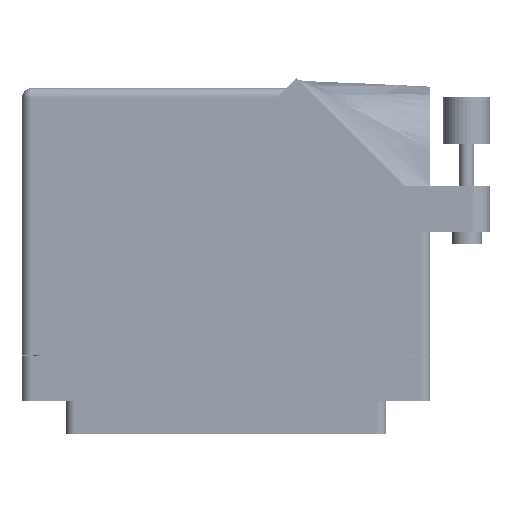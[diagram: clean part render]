
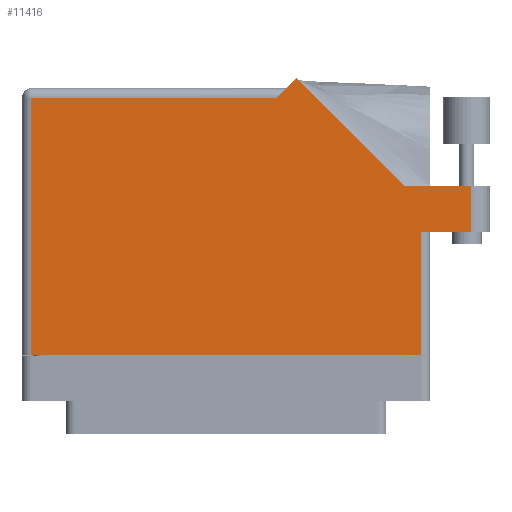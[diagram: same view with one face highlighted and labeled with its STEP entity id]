
A CAD part, front view. The second image highlights one B-rep face of the part: STEP entity #11416.
In plain terms, the highlighted face is planar.
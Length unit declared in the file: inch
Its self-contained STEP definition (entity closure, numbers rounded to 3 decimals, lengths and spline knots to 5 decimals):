
#575 = CARTESIAN_POINT ( 'NONE',  ( 1.297, 0.715, 0.617 ) ) ;
#793 = DIRECTION ( 'NONE',  ( -1., 0., 0. ) ) ;
#1383 = VERTEX_POINT ( 'NONE', #56044 ) ;
#2882 = EDGE_CURVE ( 'NONE', #39727, #57878, #27326, .T. ) ;
#3471 = ORIENTED_EDGE ( 'NONE', *, *, #36136, .T. ) ;
#3594 = VERTEX_POINT ( 'NONE', #21968 ) ;
#4617 = LINE ( 'NONE', #35553, #37606 ) ;
#5000 = DIRECTION ( 'NONE',  ( -1., 0., 0. ) ) ;
#7629 = CARTESIAN_POINT ( 'NONE',  ( -1.297, -0.1, 0.617 ) ) ;
#8923 = CARTESIAN_POINT ( 'NONE',  ( 1.19342, 1.022, 0.617 ) ) ;
#11416 = ADVANCED_FACE ( 'NONE', ( #44479 ), #49639, .F. ) ;
#13056 = VECTOR ( 'NONE', #793, 39.37008 ) ;
#13113 = LINE ( 'NONE', #18179, #72159 ) ;
#14040 = EDGE_CURVE ( 'NONE', #65003, #15289, #53946, .T. ) ;
#14169 = ORIENTED_EDGE ( 'NONE', *, *, #66457, .T. ) ;
#14201 = CARTESIAN_POINT ( 'NONE',  ( 1.297, 0.715, 0.617 ) ) ;
#15011 = CARTESIAN_POINT ( 'NONE',  ( 0.399, 1.675, 0.617 ) ) ;
#15289 = VERTEX_POINT ( 'NONE', #29542 ) ;
#16509 = ORIENTED_EDGE ( 'NONE', *, *, #23540, .T. ) ;
#18179 = CARTESIAN_POINT ( 'NONE',  ( -1.359, -0.1, 0.617 ) ) ;
#18194 = ORIENTED_EDGE ( 'NONE', *, *, #22297, .T. ) ;
#18406 = CARTESIAN_POINT ( 'NONE',  ( 1.759, 1.022, 0.617 ) ) ;
#19467 = CARTESIAN_POINT ( 'NONE',  ( 1.634, 0.715, 0.617 ) ) ;
#19882 = EDGE_LOOP ( 'NONE', ( #3471, #60425, #14169, #16509, #44811, #64625, #18194, #25845, #32673 ) ) ;
#21968 = CARTESIAN_POINT ( 'NONE',  ( 0.337, 1.613, 0.617 ) ) ;
#22297 = EDGE_CURVE ( 'NONE', #1383, #32161, #22574, .T. ) ;
#22574 = LINE ( 'NONE', #53452, #25234 ) ;
#22772 = CARTESIAN_POINT ( 'NONE',  ( 1.297, -0.1, 0.617 ) ) ;
#23540 = EDGE_CURVE ( 'NONE', #53965, #62565, #59020, .T. ) ;
#25234 = VECTOR ( 'NONE', #32179, 39.37008 ) ;
#25845 = ORIENTED_EDGE ( 'NONE', *, *, #62124, .T. ) ;
#26243 = DIRECTION ( 'NONE',  ( 1., 0., 0. ) ) ;
#26257 = VECTOR ( 'NONE', #28335, 39.37008 ) ;
#26466 = VECTOR ( 'NONE', #31413, 39.37008 ) ;
#27132 = CARTESIAN_POINT ( 'NONE',  ( 1.19342, 1.022, 0.617 ) ) ;
#27326 = LINE ( 'NONE', #14201, #26466 ) ;
#28335 = DIRECTION ( 'NONE',  ( 0., 1., 0. ) ) ;
#29542 = CARTESIAN_POINT ( 'NONE',  ( 1.634, 1.022, 0.617 ) ) ;
#31413 = DIRECTION ( 'NONE',  ( 0., 1., 0. ) ) ;
#31524 = DIRECTION ( 'NONE',  ( -0.707, -0.707, 0. ) ) ;
#32100 = CARTESIAN_POINT ( 'NONE',  ( 0.46971, 1.74571, 0.617 ) ) ;
#32161 = VERTEX_POINT ( 'NONE', #7629 ) ;
#32179 = DIRECTION ( 'NONE',  ( 0., -1., 0. ) ) ;
#32549 = VECTOR ( 'NONE', #5000, 39.37008 ) ;
#32673 = ORIENTED_EDGE ( 'NONE', *, *, #2882, .T. ) ;
#32889 = DIRECTION ( 'NONE',  ( -0.707, 0.707, 0. ) ) ;
#34887 = EDGE_CURVE ( 'NONE', #3594, #1383, #41506, .T. ) ;
#35553 = CARTESIAN_POINT ( 'NONE',  ( 1.359, 0.715, 0.617 ) ) ;
#36136 = EDGE_CURVE ( 'NONE', #57878, #65003, #4617, .T. ) ;
#36284 = LINE ( 'NONE', #18406, #13056 ) ;
#37606 = VECTOR ( 'NONE', #26243, 39.37008 ) ;
#38647 = DIRECTION ( 'NONE',  ( -1., 0., 0. ) ) ;
#39727 = VERTEX_POINT ( 'NONE', #22772 ) ;
#41506 = LINE ( 'NONE', #68891, #32549 ) ;
#44479 = FACE_OUTER_BOUND ( 'NONE', #19882, .T. ) ;
#44655 = VECTOR ( 'NONE', #32889, 39.37008 ) ;
#44811 = ORIENTED_EDGE ( 'NONE', *, *, #46215, .T. ) ;
#45711 = VECTOR ( 'NONE', #31524, 39.37008 ) ;
#46215 = EDGE_CURVE ( 'NONE', #62565, #3594, #49293, .T. ) ;
#49293 = LINE ( 'NONE', #15011, #45711 ) ;
#49639 = PLANE ( 'NONE',  #68329 ) ;
#49876 = CARTESIAN_POINT ( 'NONE',  ( -1.359, 1.675, 0.617 ) ) ;
#52678 = DIRECTION ( 'NONE',  ( 1., 0., 0. ) ) ;
#53452 = CARTESIAN_POINT ( 'NONE',  ( -1.297, -0.1, 0.617 ) ) ;
#53946 = LINE ( 'NONE', #73882, #26257 ) ;
#53965 = VERTEX_POINT ( 'NONE', #8923 ) ;
#56044 = CARTESIAN_POINT ( 'NONE',  ( -1.297, 1.613, 0.617 ) ) ;
#57878 = VERTEX_POINT ( 'NONE', #575 ) ;
#59020 = LINE ( 'NONE', #27132, #44655 ) ;
#60425 = ORIENTED_EDGE ( 'NONE', *, *, #14040, .T. ) ;
#62124 = EDGE_CURVE ( 'NONE', #32161, #39727, #13113, .T. ) ;
#62565 = VERTEX_POINT ( 'NONE', #32100 ) ;
#64625 = ORIENTED_EDGE ( 'NONE', *, *, #34887, .T. ) ;
#65003 = VERTEX_POINT ( 'NONE', #19467 ) ;
#66457 = EDGE_CURVE ( 'NONE', #15289, #53965, #36284, .T. ) ;
#68329 = AXIS2_PLACEMENT_3D ( 'NONE', #49876, #72920, #38647 ) ;
#68891 = CARTESIAN_POINT ( 'NONE',  ( -1.359, 1.613, 0.617 ) ) ;
#72159 = VECTOR ( 'NONE', #52678, 39.37008 ) ;
#72920 = DIRECTION ( 'NONE',  ( 0., 0., -1. ) ) ;
#73882 = CARTESIAN_POINT ( 'NONE',  ( 1.634, 1.022, 0.617 ) ) ;
